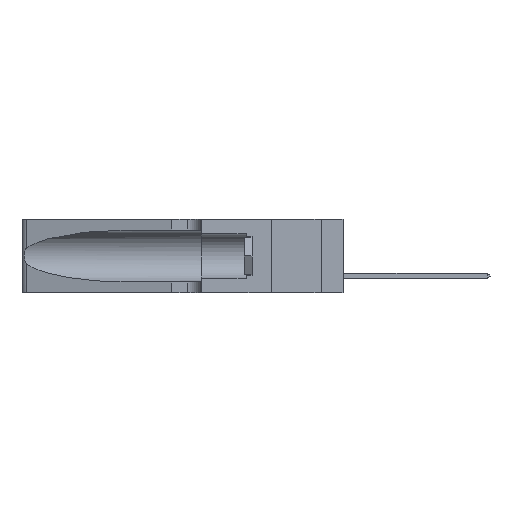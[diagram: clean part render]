
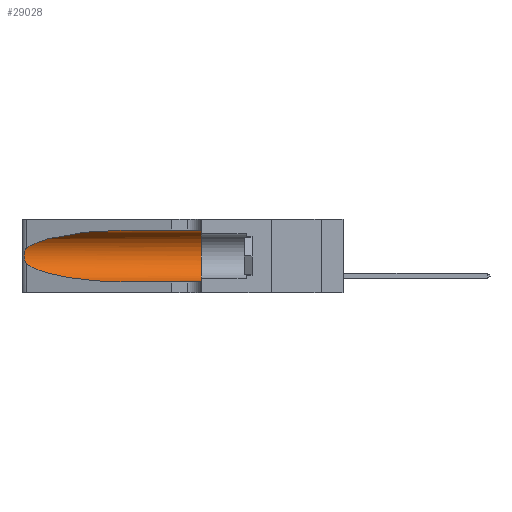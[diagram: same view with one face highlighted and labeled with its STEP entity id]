
A CAD part, left-side view. The second image highlights one B-rep face of the part: STEP entity #29028.
In plain terms, the highlighted cylindrical face has radius 3.308 mm (diameter 6.617 mm), a partial arc.
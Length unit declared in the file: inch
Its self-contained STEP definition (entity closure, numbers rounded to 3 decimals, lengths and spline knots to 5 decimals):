
#662 = B_SPLINE_CURVE_WITH_KNOTS ( 'NONE', 3,
 ( #4239, #44539, #36469, #28686, #36303, #8462, #32213, #48810, #8110, #20565, #20398, #28503, #12286, #40126 ),
 .UNSPECIFIED., .F., .F.,
 ( 4, 2, 2, 2, 2, 2, 4 ),
 ( 0., 0.00027, 0.00053, 0.00107, 0.0016, 0.00187, 0.00214 ),
 .UNSPECIFIED. ) ;
#1215 = ORIENTED_EDGE ( 'NONE', *, *, #36011, .T. ) ;
#1983 = VERTEX_POINT ( 'NONE', #48461 ) ;
#3645 = EDGE_LOOP ( 'NONE', ( #40718, #19683, #47577, #1215, #35930, #27137 ) ) ;
#4239 = CARTESIAN_POINT ( 'NONE',  ( 0.25487, 1.22718, 0.22369 ) ) ;
#4271 = CARTESIAN_POINT ( 'NONE',  ( 0.1305, 0.72297, 0.31525 ) ) ;
#4373 = LINE ( 'NONE', #35019, #17567 ) ;
#5769 = CARTESIAN_POINT ( 'NONE',  ( 0.1305, 0.35, 0.05475 ) ) ;
#5818 = CARTESIAN_POINT ( 'NONE',  ( 0.25487, 1.22718, 0.14631 ) ) ;
#6076 = CARTESIAN_POINT ( 'NONE',  ( 0.1305, 1.61858, 0.185 ) ) ;
#7481 = CARTESIAN_POINT ( 'NONE',  ( 0.25487, 1.22718, 0.14631 ) ) ;
#8110 = CARTESIAN_POINT ( 'NONE',  ( 0.26017, 1.23833, 0.17102 ) ) ;
#8462 = CARTESIAN_POINT ( 'NONE',  ( 0.26018, 1.23835, 0.19895 ) ) ;
#10459 = DIRECTION ( 'NONE',  ( 0., -1., 0. ) ) ;
#10538 = CARTESIAN_POINT ( 'NONE',  ( 0.1305, 0.72297, 0.05475 ) ) ;
#12286 = CARTESIAN_POINT ( 'NONE',  ( 0.25555, 1.22993, 0.14849 ) ) ;
#17567 = VECTOR ( 'NONE', #22334, 39.37008 ) ;
#18011 = DIRECTION ( 'NONE',  ( 0., 0., -1. ) ) ;
#18836 = AXIS2_PLACEMENT_3D ( 'NONE', #23104, #27145, #42996 ) ;
#18988 = VERTEX_POINT ( 'NONE', #32012 ) ;
#19117 = CYLINDRICAL_SURFACE ( 'NONE', #49866, 0.13025 ) ;
#19683 = ORIENTED_EDGE ( 'NONE', *, *, #32827, .T. ) ;
#19729 = EDGE_CURVE ( 'NONE', #18988, #46060, #25641, .T. ) ;
#19981 = EDGE_CURVE ( 'NONE', #26949, #1983, #30998, .T. ) ;
#20398 = CARTESIAN_POINT ( 'NONE',  ( 0.25789, 1.23486, 0.15765 ) ) ;
#20565 = CARTESIAN_POINT ( 'NONE',  ( 0.25856, 1.23593, 0.16098 ) ) ;
#22334 = DIRECTION ( 'NONE',  ( 0., -1., 0. ) ) ;
#23104 = CARTESIAN_POINT ( 'NONE',  ( 0.1305, 0.35, 0.185 ) ) ;
#24870 =( BOUNDED_CURVE ( )  B_SPLINE_CURVE ( 3, ( #5818, #33275, #25542, #41533 ),
 .UNSPECIFIED., .F., .F. ) 
 B_SPLINE_CURVE_WITH_KNOTS ( ( 4, 4 ),
 ( 3.44316, 4.71239 ),
 .UNSPECIFIED. ) 
 CURVE ( )  GEOMETRIC_REPRESENTATION_ITEM ( )  RATIONAL_B_SPLINE_CURVE ( ( 1., 0.87, 0.87, 1. ) ) 
 REPRESENTATION_ITEM ( '' )  );
#25542 = CARTESIAN_POINT ( 'NONE',  ( 0.18966, 0.96281, 0.05475 ) ) ;
#25641 = CIRCLE ( 'NONE', #18836, 0.13025 ) ;
#26949 = VERTEX_POINT ( 'NONE', #50167 ) ;
#27116 = LINE ( 'NONE', #30793, #37840 ) ;
#27137 = ORIENTED_EDGE ( 'NONE', *, *, #47517, .F. ) ;
#27145 = DIRECTION ( 'NONE',  ( 0., 1., 0. ) ) ;
#28503 = CARTESIAN_POINT ( 'NONE',  ( 0.25639, 1.23186, 0.15144 ) ) ;
#28686 = CARTESIAN_POINT ( 'NONE',  ( 0.25787, 1.23484, 0.2124 ) ) ;
#29028 = ADVANCED_FACE ( 'NONE', ( #31085 ), #19117, .F. ) ;
#29234 = CARTESIAN_POINT ( 'NONE',  ( 0.2373, 1.15595, 0.28018 ) ) ;
#30793 = CARTESIAN_POINT ( 'NONE',  ( 0.1305, 1.61858, 0.31525 ) ) ;
#30998 =( BOUNDED_CURVE ( )  B_SPLINE_CURVE ( 3, ( #4271, #52219, #29234, #37196 ),
 .UNSPECIFIED., .F., .F. ) 
 B_SPLINE_CURVE_WITH_KNOTS ( ( 4, 4 ),
 ( 1.5708, 2.84003 ),
 .UNSPECIFIED. ) 
 CURVE ( )  GEOMETRIC_REPRESENTATION_ITEM ( )  RATIONAL_B_SPLINE_CURVE ( ( 1., 0.87, 0.87, 1. ) ) 
 REPRESENTATION_ITEM ( '' )  );
#31085 = FACE_OUTER_BOUND ( 'NONE', #3645, .T. ) ;
#32012 = CARTESIAN_POINT ( 'NONE',  ( 0.1305, 0.35, 0.31525 ) ) ;
#32213 = CARTESIAN_POINT ( 'NONE',  ( 0.26075, 1.23896, 0.19203 ) ) ;
#32827 = EDGE_CURVE ( 'NONE', #1983, #38105, #662, .T. ) ;
#33275 = CARTESIAN_POINT ( 'NONE',  ( 0.2373, 1.15595, 0.08982 ) ) ;
#35019 = CARTESIAN_POINT ( 'NONE',  ( 0.1305, 1.61858, 0.05475 ) ) ;
#35930 = ORIENTED_EDGE ( 'NONE', *, *, #19729, .F. ) ;
#36011 = EDGE_CURVE ( 'NONE', #36081, #46060, #4373, .T. ) ;
#36081 = VERTEX_POINT ( 'NONE', #10538 ) ;
#36303 = CARTESIAN_POINT ( 'NONE',  ( 0.25854, 1.2359, 0.20912 ) ) ;
#36469 = CARTESIAN_POINT ( 'NONE',  ( 0.25639, 1.23184, 0.21858 ) ) ;
#37196 = CARTESIAN_POINT ( 'NONE',  ( 0.25487, 1.22718, 0.22369 ) ) ;
#37840 = VECTOR ( 'NONE', #38557, 39.37008 ) ;
#38105 = VERTEX_POINT ( 'NONE', #7481 ) ;
#38557 = DIRECTION ( 'NONE',  ( 0., -1., 0. ) ) ;
#40126 = CARTESIAN_POINT ( 'NONE',  ( 0.25487, 1.22718, 0.14631 ) ) ;
#40718 = ORIENTED_EDGE ( 'NONE', *, *, #19981, .T. ) ;
#41533 = CARTESIAN_POINT ( 'NONE',  ( 0.1305, 0.72297, 0.05475 ) ) ;
#42996 = DIRECTION ( 'NONE',  ( 0., 0., 1. ) ) ;
#44539 = CARTESIAN_POINT ( 'NONE',  ( 0.25555, 1.22994, 0.2215 ) ) ;
#46060 = VERTEX_POINT ( 'NONE', #5769 ) ;
#47517 = EDGE_CURVE ( 'NONE', #26949, #18988, #27116, .T. ) ;
#47577 = ORIENTED_EDGE ( 'NONE', *, *, #49356, .T. ) ;
#48461 = CARTESIAN_POINT ( 'NONE',  ( 0.25487, 1.22718, 0.22369 ) ) ;
#48810 = CARTESIAN_POINT ( 'NONE',  ( 0.26075, 1.23896, 0.178 ) ) ;
#49356 = EDGE_CURVE ( 'NONE', #38105, #36081, #24870, .T. ) ;
#49866 = AXIS2_PLACEMENT_3D ( 'NONE', #6076, #10459, #18011 ) ;
#50167 = CARTESIAN_POINT ( 'NONE',  ( 0.1305, 0.72297, 0.31525 ) ) ;
#52219 = CARTESIAN_POINT ( 'NONE',  ( 0.18966, 0.96281, 0.31525 ) ) ;
